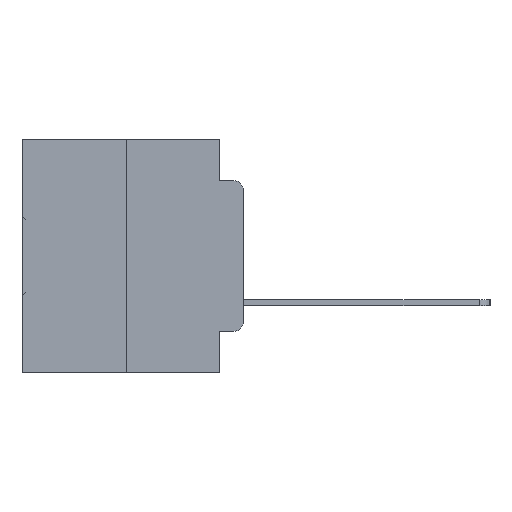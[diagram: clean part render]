
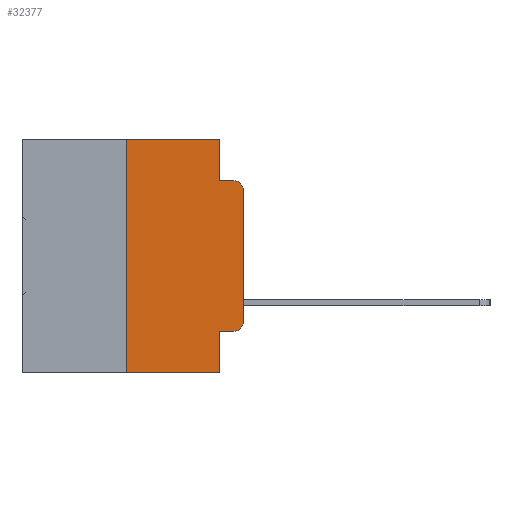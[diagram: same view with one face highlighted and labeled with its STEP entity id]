
A CAD part, left-side view. The second image highlights one B-rep face of the part: STEP entity #32377.
In plain terms, the highlighted planar face has unit normal (-1, 0, 0).
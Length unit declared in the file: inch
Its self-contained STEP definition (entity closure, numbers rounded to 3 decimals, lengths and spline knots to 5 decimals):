
#160 = VERTEX_POINT ( 'NONE', #9600 ) ;
#340 = ORIENTED_EDGE ( 'NONE', *, *, #15498, .T. ) ;
#364 = CARTESIAN_POINT ( 'NONE',  ( 0., 0.02, -0.4115 ) ) ;
#964 = EDGE_CURVE ( 'NONE', #27074, #18912, #21099, .T. ) ;
#1425 = DIRECTION ( 'NONE',  ( -1., 0., 0. ) ) ;
#1562 = ORIENTED_EDGE ( 'NONE', *, *, #1915, .F. ) ;
#1910 = DIRECTION ( 'NONE',  ( 0., 0., 1. ) ) ;
#1915 = EDGE_CURVE ( 'NONE', #32153, #31905, #14158, .T. ) ;
#3253 = EDGE_CURVE ( 'NONE', #27574, #17806, #26124, .T. ) ;
#3630 = DIRECTION ( 'NONE',  ( 0., 0., -1. ) ) ;
#4460 = VERTEX_POINT ( 'NONE', #364 ) ;
#5035 = CARTESIAN_POINT ( 'NONE',  ( 0., 0.25, -0.5 ) ) ;
#5168 = CARTESIAN_POINT ( 'NONE',  ( 0., 0.051, -0.4115 ) ) ;
#5940 = CARTESIAN_POINT ( 'NONE',  ( 0., 0.02, -0.1085 ) ) ;
#5979 = ORIENTED_EDGE ( 'NONE', *, *, #22050, .F. ) ;
#7367 = VECTOR ( 'NONE', #10003, 39.37008 ) ;
#7683 = CARTESIAN_POINT ( 'NONE',  ( 0., 0.051, -0.0885 ) ) ;
#8368 = DIRECTION ( 'NONE',  ( 0., 0., -1. ) ) ;
#8548 = DIRECTION ( 'NONE',  ( 0., 0., -1. ) ) ;
#8779 = CARTESIAN_POINT ( 'NONE',  ( 0., 0.473, 0. ) ) ;
#8913 = CARTESIAN_POINT ( 'NONE',  ( 0., 0.051, 0. ) ) ;
#8976 = CARTESIAN_POINT ( 'NONE',  ( 0., 0.02, -0.0885 ) ) ;
#9454 = CARTESIAN_POINT ( 'NONE',  ( 0., 0., 0. ) ) ;
#9600 = CARTESIAN_POINT ( 'NONE',  ( 0., 0., -0.1085 ) ) ;
#10003 = DIRECTION ( 'NONE',  ( 0., -1., 0. ) ) ;
#10951 = VERTEX_POINT ( 'NONE', #5035 ) ;
#11189 = LINE ( 'NONE', #26977, #16472 ) ;
#11238 = ORIENTED_EDGE ( 'NONE', *, *, #25487, .T. ) ;
#11391 = AXIS2_PLACEMENT_3D ( 'NONE', #5940, #23995, #8548 ) ;
#12052 = ORIENTED_EDGE ( 'NONE', *, *, #3253, .F. ) ;
#12574 = VECTOR ( 'NONE', #32839, 39.37008 ) ;
#12587 = EDGE_CURVE ( 'NONE', #10951, #31905, #11189, .T. ) ;
#12974 = LINE ( 'NONE', #14773, #19069 ) ;
#13186 = LINE ( 'NONE', #23822, #26834 ) ;
#13346 = VECTOR ( 'NONE', #3630, 39.37008 ) ;
#13706 = FACE_OUTER_BOUND ( 'NONE', #28386, .T. ) ;
#13794 = AXIS2_PLACEMENT_3D ( 'NONE', #8779, #13976, #31844 ) ;
#13976 = DIRECTION ( 'NONE',  ( 1., 0., 0. ) ) ;
#14158 = LINE ( 'NONE', #21699, #13346 ) ;
#14195 = VECTOR ( 'NONE', #27436, 39.37008 ) ;
#14486 = ORIENTED_EDGE ( 'NONE', *, *, #15121, .F. ) ;
#14773 = CARTESIAN_POINT ( 'NONE',  ( 0., 0.25, 0. ) ) ;
#15121 = EDGE_CURVE ( 'NONE', #10951, #27074, #12974, .T. ) ;
#15498 = EDGE_CURVE ( 'NONE', #4460, #18033, #16177, .T. ) ;
#16177 = CIRCLE ( 'NONE', #27628, 0.02 ) ;
#16472 = VECTOR ( 'NONE', #19442, 39.37008 ) ;
#16918 = CARTESIAN_POINT ( 'NONE',  ( 0., 0.02, -0.3915 ) ) ;
#17806 = VERTEX_POINT ( 'NONE', #8976 ) ;
#18033 = VERTEX_POINT ( 'NONE', #28289 ) ;
#18119 = DIRECTION ( 'NONE',  ( 0., -1., 0. ) ) ;
#18414 = CARTESIAN_POINT ( 'NONE',  ( 0., 0.051, -0.0885 ) ) ;
#18912 = VERTEX_POINT ( 'NONE', #8913 ) ;
#19069 = VECTOR ( 'NONE', #1910, 39.37008 ) ;
#19442 = DIRECTION ( 'NONE',  ( 0., -1., 0. ) ) ;
#19534 = DIRECTION ( 'NONE',  ( 0., 0., -1. ) ) ;
#19780 = ORIENTED_EDGE ( 'NONE', *, *, #964, .F. ) ;
#20179 = VECTOR ( 'NONE', #18119, 39.37008 ) ;
#20323 = CARTESIAN_POINT ( 'NONE',  ( 0., 0.051, -0.4115 ) ) ;
#21099 = LINE ( 'NONE', #30493, #7367 ) ;
#21439 = PLANE ( 'NONE',  #13794 ) ;
#21699 = CARTESIAN_POINT ( 'NONE',  ( 0., 0.051, 0. ) ) ;
#22050 = EDGE_CURVE ( 'NONE', #18912, #27574, #13186, .T. ) ;
#23822 = CARTESIAN_POINT ( 'NONE',  ( 0., 0.051, 0. ) ) ;
#23995 = DIRECTION ( 'NONE',  ( -1., 0., 0. ) ) ;
#24931 = ORIENTED_EDGE ( 'NONE', *, *, #30561, .T. ) ;
#25487 = EDGE_CURVE ( 'NONE', #18033, #160, #28608, .T. ) ;
#26124 = LINE ( 'NONE', #7683, #20179 ) ;
#26232 = LINE ( 'NONE', #20323, #12574 ) ;
#26834 = VECTOR ( 'NONE', #8368, 39.37008 ) ;
#26977 = CARTESIAN_POINT ( 'NONE',  ( 0., 0.473, -0.5 ) ) ;
#27074 = VERTEX_POINT ( 'NONE', #31172 ) ;
#27436 = DIRECTION ( 'NONE',  ( 0., 0., 1. ) ) ;
#27574 = VERTEX_POINT ( 'NONE', #18414 ) ;
#27628 = AXIS2_PLACEMENT_3D ( 'NONE', #16918, #1425, #19534 ) ;
#28126 = ORIENTED_EDGE ( 'NONE', *, *, #12587, .T. ) ;
#28289 = CARTESIAN_POINT ( 'NONE',  ( 0., 0., -0.3915 ) ) ;
#28386 = EDGE_LOOP ( 'NONE', ( #11238, #24931, #12052, #5979, #19780, #14486, #28126, #1562, #29678, #340 ) ) ;
#28608 = LINE ( 'NONE', #9454, #14195 ) ;
#29678 = ORIENTED_EDGE ( 'NONE', *, *, #30073, .T. ) ;
#29757 = CARTESIAN_POINT ( 'NONE',  ( 0., 0.051, -0.5 ) ) ;
#30073 = EDGE_CURVE ( 'NONE', #32153, #4460, #26232, .T. ) ;
#30493 = CARTESIAN_POINT ( 'NONE',  ( 0., 0.473, 0. ) ) ;
#30561 = EDGE_CURVE ( 'NONE', #160, #17806, #31323, .T. ) ;
#31172 = CARTESIAN_POINT ( 'NONE',  ( 0., 0.25, 0. ) ) ;
#31323 = CIRCLE ( 'NONE', #11391, 0.02 ) ;
#31844 = DIRECTION ( 'NONE',  ( 0., 0., -1. ) ) ;
#31905 = VERTEX_POINT ( 'NONE', #29757 ) ;
#32153 = VERTEX_POINT ( 'NONE', #5168 ) ;
#32377 = ADVANCED_FACE ( 'NONE', ( #13706 ), #21439, .F. ) ;
#32839 = DIRECTION ( 'NONE',  ( 0., -1., 0. ) ) ;
